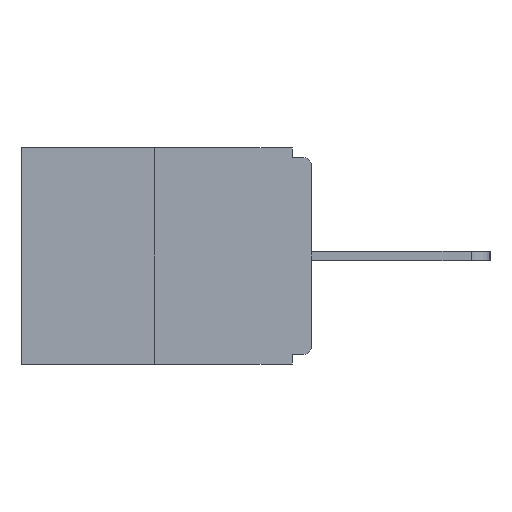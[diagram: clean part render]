
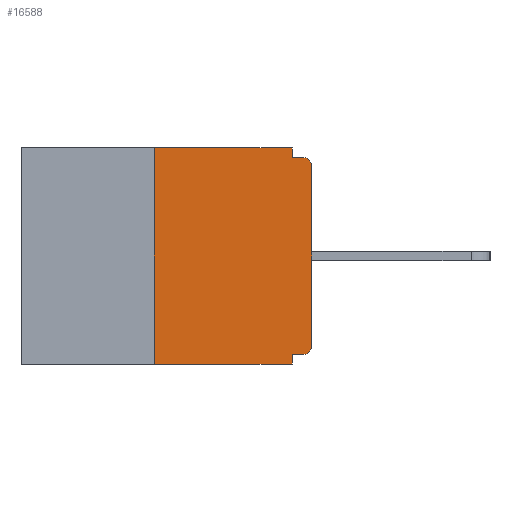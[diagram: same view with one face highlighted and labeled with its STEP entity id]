
A CAD part, left-side view. The second image highlights one B-rep face of the part: STEP entity #16588.
In plain terms, the highlighted planar face has unit normal (-1, 0, 0).
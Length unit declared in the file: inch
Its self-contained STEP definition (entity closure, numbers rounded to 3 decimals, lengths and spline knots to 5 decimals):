
#350 = AXIS2_PLACEMENT_3D ( 'NONE', #18468, #14598, #12445 ) ;
#448 = VERTEX_POINT ( 'NONE', #1958 ) ;
#608 = LINE ( 'NONE', #8801, #11701 ) ;
#877 = LINE ( 'NONE', #15941, #8233 ) ;
#1083 = LINE ( 'NONE', #7498, #12189 ) ;
#1255 = EDGE_LOOP ( 'NONE', ( #12470, #16645, #5774, #13380, #10078, #17907, #7133, #15181, #4188, #8984 ) ) ;
#1740 = EDGE_CURVE ( 'NONE', #2266, #17437, #1083, .T. ) ;
#1775 = DIRECTION ( 'NONE',  ( -1., 0., 0. ) ) ;
#1958 = CARTESIAN_POINT ( 'NONE',  ( 0., 0.015, -0.328 ) ) ;
#2016 = CARTESIAN_POINT ( 'NONE',  ( 0., 0., -0.03 ) ) ;
#2076 = LINE ( 'NONE', #12373, #14059 ) ;
#2266 = VERTEX_POINT ( 'NONE', #2624 ) ;
#2624 = CARTESIAN_POINT ( 'NONE',  ( 0., 0.25, 0. ) ) ;
#2740 = VECTOR ( 'NONE', #4987, 39.37008 ) ;
#2757 = CARTESIAN_POINT ( 'NONE',  ( 0., 0.031, -0.015 ) ) ;
#3164 = CARTESIAN_POINT ( 'NONE',  ( 0., 0.031, 0. ) ) ;
#3767 = DIRECTION ( 'NONE',  ( 0., 0., -1. ) ) ;
#3859 = PLANE ( 'NONE',  #14783 ) ;
#4057 = DIRECTION ( 'NONE',  ( 0., 0., 1. ) ) ;
#4188 = ORIENTED_EDGE ( 'NONE', *, *, #14622, .F. ) ;
#4557 = EDGE_CURVE ( 'NONE', #13062, #16440, #877, .T. ) ;
#4689 = VERTEX_POINT ( 'NONE', #16449 ) ;
#4987 = DIRECTION ( 'NONE',  ( 0., 1., 0. ) ) ;
#5102 = FACE_OUTER_BOUND ( 'NONE', #1255, .T. ) ;
#5231 = CARTESIAN_POINT ( 'NONE',  ( 0., 0., -0.313 ) ) ;
#5353 = DIRECTION ( 'NONE',  ( 0., -1., 0. ) ) ;
#5774 = ORIENTED_EDGE ( 'NONE', *, *, #11837, .T. ) ;
#6092 = LINE ( 'NONE', #8049, #13207 ) ;
#6151 = EDGE_CURVE ( 'NONE', #16440, #11406, #12140, .T. ) ;
#6692 = LINE ( 'NONE', #15368, #14248 ) ;
#6808 = CARTESIAN_POINT ( 'NONE',  ( 0., 0.46, 0. ) ) ;
#7133 = ORIENTED_EDGE ( 'NONE', *, *, #4557, .T. ) ;
#7415 = EDGE_CURVE ( 'NONE', #17437, #8983, #6092, .T. ) ;
#7498 = CARTESIAN_POINT ( 'NONE',  ( 0., 0.46, 0. ) ) ;
#7530 = LINE ( 'NONE', #12637, #11291 ) ;
#7859 = CARTESIAN_POINT ( 'NONE',  ( 0., 0., -0.328 ) ) ;
#8049 = CARTESIAN_POINT ( 'NONE',  ( 0., 0.031, 0. ) ) ;
#8094 = DIRECTION ( 'NONE',  ( 0., 0., -1. ) ) ;
#8233 = VECTOR ( 'NONE', #16124, 39.37008 ) ;
#8263 = DIRECTION ( 'NONE',  ( 0., 0., -1. ) ) ;
#8574 = CARTESIAN_POINT ( 'NONE',  ( 0., 0.015, -0.015 ) ) ;
#8790 = CARTESIAN_POINT ( 'NONE',  ( 0., 0.031, -0.328 ) ) ;
#8801 = CARTESIAN_POINT ( 'NONE',  ( 0., 0., -0.015 ) ) ;
#8983 = VERTEX_POINT ( 'NONE', #2757 ) ;
#8984 = ORIENTED_EDGE ( 'NONE', *, *, #7415, .F. ) ;
#10078 = ORIENTED_EDGE ( 'NONE', *, *, #12964, .F. ) ;
#10203 = DIRECTION ( 'NONE',  ( 0., -1., 0. ) ) ;
#10548 = CARTESIAN_POINT ( 'NONE',  ( 0., 0.015, -0.313 ) ) ;
#11163 = CARTESIAN_POINT ( 'NONE',  ( 0., 0.25, -0.343 ) ) ;
#11216 = EDGE_CURVE ( 'NONE', #12677, #4689, #2076, .T. ) ;
#11291 = VECTOR ( 'NONE', #4057, 39.37008 ) ;
#11406 = VERTEX_POINT ( 'NONE', #8574 ) ;
#11701 = VECTOR ( 'NONE', #10203, 39.37008 ) ;
#11837 = EDGE_CURVE ( 'NONE', #17743, #4689, #6692, .T. ) ;
#11933 = DIRECTION ( 'NONE',  ( 0., 0., -1. ) ) ;
#12140 = CIRCLE ( 'NONE', #350, 0.015 ) ;
#12189 = VECTOR ( 'NONE', #13722, 39.37008 ) ;
#12373 = CARTESIAN_POINT ( 'NONE',  ( 0., 0.031, -0.343 ) ) ;
#12445 = DIRECTION ( 'NONE',  ( 0., 0., -1. ) ) ;
#12470 = ORIENTED_EDGE ( 'NONE', *, *, #1740, .F. ) ;
#12637 = CARTESIAN_POINT ( 'NONE',  ( 0., 0.25, 0. ) ) ;
#12677 = VERTEX_POINT ( 'NONE', #8790 ) ;
#12964 = EDGE_CURVE ( 'NONE', #448, #12677, #17874, .T. ) ;
#13062 = VERTEX_POINT ( 'NONE', #5231 ) ;
#13207 = VECTOR ( 'NONE', #8094, 39.37008 ) ;
#13380 = ORIENTED_EDGE ( 'NONE', *, *, #11216, .F. ) ;
#13722 = DIRECTION ( 'NONE',  ( 0., -1., 0. ) ) ;
#14059 = VECTOR ( 'NONE', #3767, 39.37008 ) ;
#14248 = VECTOR ( 'NONE', #5353, 39.37008 ) ;
#14598 = DIRECTION ( 'NONE',  ( -1., 0., 0. ) ) ;
#14622 = EDGE_CURVE ( 'NONE', #8983, #11406, #608, .T. ) ;
#14655 = AXIS2_PLACEMENT_3D ( 'NONE', #10548, #1775, #11933 ) ;
#14783 = AXIS2_PLACEMENT_3D ( 'NONE', #6808, #16690, #8263 ) ;
#15181 = ORIENTED_EDGE ( 'NONE', *, *, #6151, .T. ) ;
#15368 = CARTESIAN_POINT ( 'NONE',  ( 0., 0.46, -0.343 ) ) ;
#15941 = CARTESIAN_POINT ( 'NONE',  ( 0., 0., 0. ) ) ;
#16007 = CIRCLE ( 'NONE', #14655, 0.015 ) ;
#16124 = DIRECTION ( 'NONE',  ( 0., 0., 1. ) ) ;
#16440 = VERTEX_POINT ( 'NONE', #2016 ) ;
#16449 = CARTESIAN_POINT ( 'NONE',  ( 0., 0.031, -0.343 ) ) ;
#16588 = ADVANCED_FACE ( 'NONE', ( #5102 ), #3859, .F. ) ;
#16645 = ORIENTED_EDGE ( 'NONE', *, *, #18315, .F. ) ;
#16690 = DIRECTION ( 'NONE',  ( 1., 0., 0. ) ) ;
#17437 = VERTEX_POINT ( 'NONE', #3164 ) ;
#17478 = EDGE_CURVE ( 'NONE', #448, #13062, #16007, .T. ) ;
#17743 = VERTEX_POINT ( 'NONE', #11163 ) ;
#17874 = LINE ( 'NONE', #7859, #2740 ) ;
#17907 = ORIENTED_EDGE ( 'NONE', *, *, #17478, .T. ) ;
#18315 = EDGE_CURVE ( 'NONE', #17743, #2266, #7530, .T. ) ;
#18468 = CARTESIAN_POINT ( 'NONE',  ( 0., 0.015, -0.03 ) ) ;
